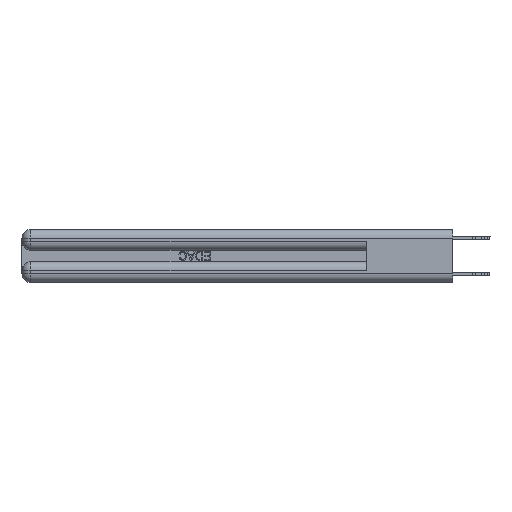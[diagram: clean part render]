
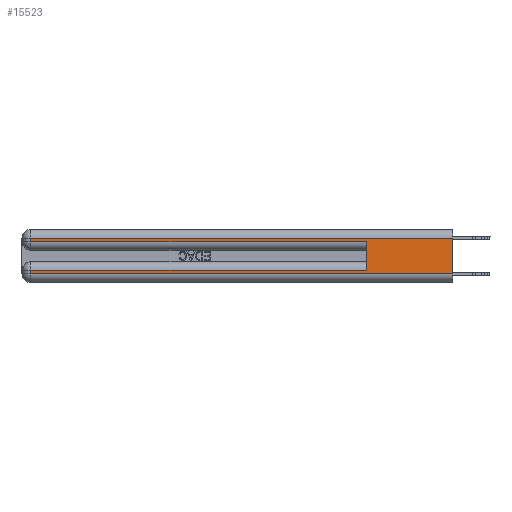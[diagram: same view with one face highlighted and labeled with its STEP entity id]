
A CAD part, left-side view. The second image highlights one B-rep face of the part: STEP entity #15523.
In plain terms, the highlighted planar face has unit normal (-1, 0, 0).
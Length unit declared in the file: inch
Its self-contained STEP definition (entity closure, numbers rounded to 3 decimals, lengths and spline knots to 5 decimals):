
#96 = VECTOR ( 'NONE', #33647, 39.37008 ) ;
#372 = CARTESIAN_POINT ( 'NONE',  ( 0., 0., 0.06 ) ) ;
#1575 = CARTESIAN_POINT ( 'NONE',  ( 0., 0., 0.37 ) ) ;
#1809 = DIRECTION ( 'NONE',  ( 0., 1., 0. ) ) ;
#1873 = CARTESIAN_POINT ( 'NONE',  ( 0., 0., 0.285 ) ) ;
#2732 = EDGE_CURVE ( 'NONE', #20110, #5853, #36087, .T. ) ;
#3233 = CARTESIAN_POINT ( 'NONE',  ( 0., 0.6, 0.085 ) ) ;
#3520 = VECTOR ( 'NONE', #21543, 39.37008 ) ;
#5144 = ORIENTED_EDGE ( 'NONE', *, *, #27508, .T. ) ;
#5853 = VERTEX_POINT ( 'NONE', #6373 ) ;
#6373 = CARTESIAN_POINT ( 'NONE',  ( 0., 0.6, 0.285 ) ) ;
#6840 = EDGE_CURVE ( 'NONE', #12367, #5853, #24344, .T. ) ;
#6849 = FACE_OUTER_BOUND ( 'NONE', #24034, .T. ) ;
#7219 = ORIENTED_EDGE ( 'NONE', *, *, #6840, .F. ) ;
#7581 = DIRECTION ( 'NONE',  ( 1., 0., 0. ) ) ;
#7658 = DIRECTION ( 'NONE',  ( 0., 1., 0. ) ) ;
#7874 = VERTEX_POINT ( 'NONE', #22871 ) ;
#9236 = LINE ( 'NONE', #32361, #37044 ) ;
#9898 = EDGE_CURVE ( 'NONE', #12367, #7874, #9236, .T. ) ;
#10414 = DIRECTION ( 'NONE',  ( 0., 0., 1. ) ) ;
#11034 = LINE ( 'NONE', #31157, #27120 ) ;
#11597 = ORIENTED_EDGE ( 'NONE', *, *, #16554, .T. ) ;
#11626 = VERTEX_POINT ( 'NONE', #26139 ) ;
#12367 = VERTEX_POINT ( 'NONE', #3233 ) ;
#15523 = ADVANCED_FACE ( 'NONE', ( #6849 ), #18331, .F. ) ;
#16554 = EDGE_CURVE ( 'NONE', #11626, #29630, #16669, .T. ) ;
#16669 = LINE ( 'NONE', #18746, #34564 ) ;
#16823 = ORIENTED_EDGE ( 'NONE', *, *, #28030, .T. ) ;
#17773 = VERTEX_POINT ( 'NONE', #372 ) ;
#18331 = PLANE ( 'NONE',  #30900 ) ;
#18746 = CARTESIAN_POINT ( 'NONE',  ( 0., 0., 0.31 ) ) ;
#18756 = LINE ( 'NONE', #24027, #23499 ) ;
#18882 = CARTESIAN_POINT ( 'NONE',  ( 0., 0.6, 0.145 ) ) ;
#20110 = VERTEX_POINT ( 'NONE', #26543 ) ;
#21543 = DIRECTION ( 'NONE',  ( 0., 0., -1. ) ) ;
#22104 = LINE ( 'NONE', #33384, #3520 ) ;
#22387 = VECTOR ( 'NONE', #32537, 39.37008 ) ;
#22626 = EDGE_CURVE ( 'NONE', #29630, #20110, #22104, .T. ) ;
#22871 = CARTESIAN_POINT ( 'NONE',  ( 0., 2.94, 0.085 ) ) ;
#23499 = VECTOR ( 'NONE', #26849, 39.37008 ) ;
#24027 = CARTESIAN_POINT ( 'NONE',  ( 0., 0., 0.37 ) ) ;
#24034 = EDGE_LOOP ( 'NONE', ( #35467, #11597, #36247, #26613, #7219, #28857, #5144, #16823 ) ) ;
#24344 = LINE ( 'NONE', #18882, #25238 ) ;
#24452 = CARTESIAN_POINT ( 'NONE',  ( 0., 2.94, 0.37 ) ) ;
#25238 = VECTOR ( 'NONE', #10414, 39.37008 ) ;
#26139 = CARTESIAN_POINT ( 'NONE',  ( 0., 0., 0.31 ) ) ;
#26267 = CARTESIAN_POINT ( 'NONE',  ( 0., 2.94, 0.31 ) ) ;
#26543 = CARTESIAN_POINT ( 'NONE',  ( 0., 2.94, 0.285 ) ) ;
#26613 = ORIENTED_EDGE ( 'NONE', *, *, #2732, .T. ) ;
#26849 = DIRECTION ( 'NONE',  ( 0., 0., -1. ) ) ;
#27120 = VECTOR ( 'NONE', #33414, 39.37008 ) ;
#27508 = EDGE_CURVE ( 'NONE', #7874, #35378, #35345, .T. ) ;
#27879 = EDGE_CURVE ( 'NONE', #11626, #17773, #18756, .T. ) ;
#28030 = EDGE_CURVE ( 'NONE', #35378, #17773, #11034, .T. ) ;
#28857 = ORIENTED_EDGE ( 'NONE', *, *, #9898, .T. ) ;
#29630 = VERTEX_POINT ( 'NONE', #26267 ) ;
#30345 = DIRECTION ( 'NONE',  ( 0., 0., -1. ) ) ;
#30900 = AXIS2_PLACEMENT_3D ( 'NONE', #1575, #7581, #30345 ) ;
#31157 = CARTESIAN_POINT ( 'NONE',  ( 0., 0., 0.06 ) ) ;
#32361 = CARTESIAN_POINT ( 'NONE',  ( 0., 0., 0.085 ) ) ;
#32537 = DIRECTION ( 'NONE',  ( 0., 0., -1. ) ) ;
#32992 = CARTESIAN_POINT ( 'NONE',  ( 0., 2.94, 0.06 ) ) ;
#33384 = CARTESIAN_POINT ( 'NONE',  ( 0., 2.94, 0.37 ) ) ;
#33414 = DIRECTION ( 'NONE',  ( 0., -1., 0. ) ) ;
#33647 = DIRECTION ( 'NONE',  ( 0., -1., 0. ) ) ;
#34564 = VECTOR ( 'NONE', #1809, 39.37008 ) ;
#35345 = LINE ( 'NONE', #24452, #22387 ) ;
#35378 = VERTEX_POINT ( 'NONE', #32992 ) ;
#35467 = ORIENTED_EDGE ( 'NONE', *, *, #27879, .F. ) ;
#36087 = LINE ( 'NONE', #1873, #96 ) ;
#36247 = ORIENTED_EDGE ( 'NONE', *, *, #22626, .T. ) ;
#37044 = VECTOR ( 'NONE', #7658, 39.37008 ) ;
